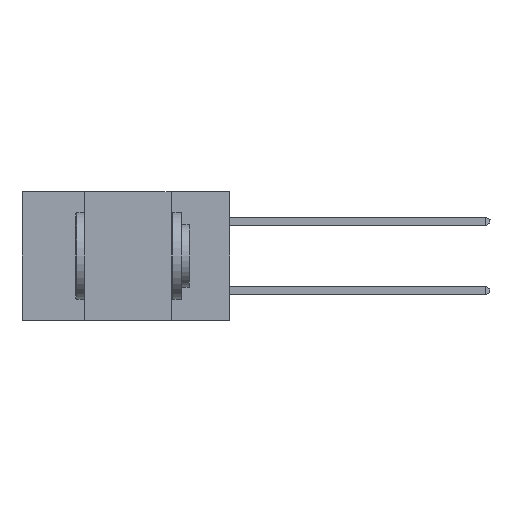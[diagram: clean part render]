
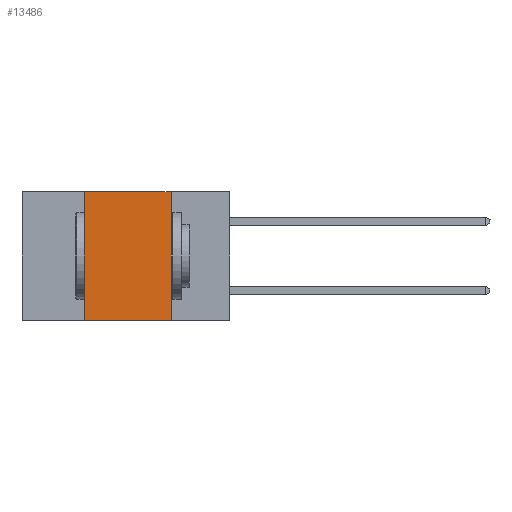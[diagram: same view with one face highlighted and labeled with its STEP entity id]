
A CAD part, left-side view. The second image highlights one B-rep face of the part: STEP entity #13486.
In plain terms, the highlighted planar face has unit normal (-1, 0, 0).
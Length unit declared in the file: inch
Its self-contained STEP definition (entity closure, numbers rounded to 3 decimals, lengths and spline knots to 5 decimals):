
#915 = LINE ( 'NONE', #7166, #13676 ) ;
#999 = FACE_OUTER_BOUND ( 'NONE', #6339, .T. ) ;
#1036 = DIRECTION ( 'NONE',  ( 0., -1., 0. ) ) ;
#2089 = DIRECTION ( 'NONE',  ( 0., 0., -1. ) ) ;
#2155 = DIRECTION ( 'NONE',  ( 1., 0., 0. ) ) ;
#2816 = VERTEX_POINT ( 'NONE', #6653 ) ;
#3292 = VECTOR ( 'NONE', #17894, 39.37008 ) ;
#3783 = EDGE_CURVE ( 'NONE', #2816, #4053, #14936, .T. ) ;
#3933 = CARTESIAN_POINT ( 'NONE',  ( 0., 0.17, 0. ) ) ;
#4053 = VERTEX_POINT ( 'NONE', #14711 ) ;
#5530 = ORIENTED_EDGE ( 'NONE', *, *, #3783, .T. ) ;
#6339 = EDGE_LOOP ( 'NONE', ( #7237, #18090, #9268, #5530 ) ) ;
#6498 = CARTESIAN_POINT ( 'NONE',  ( 0., 0.6, 0. ) ) ;
#6505 = EDGE_CURVE ( 'NONE', #9439, #10414, #10707, .T. ) ;
#6653 = CARTESIAN_POINT ( 'NONE',  ( 0., 0.42, -0.37 ) ) ;
#7166 = CARTESIAN_POINT ( 'NONE',  ( 0., 0.42, 0. ) ) ;
#7177 = LINE ( 'NONE', #18580, #16871 ) ;
#7233 = DIRECTION ( 'NONE',  ( 0., 0., 1. ) ) ;
#7237 = ORIENTED_EDGE ( 'NONE', *, *, #12607, .F. ) ;
#7510 = CARTESIAN_POINT ( 'NONE',  ( 0., 0.6, -0.37 ) ) ;
#9268 = ORIENTED_EDGE ( 'NONE', *, *, #20743, .F. ) ;
#9439 = VERTEX_POINT ( 'NONE', #13994 ) ;
#10278 = CARTESIAN_POINT ( 'NONE',  ( 0., 0.6, 0. ) ) ;
#10414 = VERTEX_POINT ( 'NONE', #3933 ) ;
#10707 = LINE ( 'NONE', #6498, #3292 ) ;
#12607 = EDGE_CURVE ( 'NONE', #10414, #4053, #7177, .T. ) ;
#13486 = ADVANCED_FACE ( 'NONE', ( #999 ), #19961, .F. ) ;
#13676 = VECTOR ( 'NONE', #7233, 39.37008 ) ;
#13994 = CARTESIAN_POINT ( 'NONE',  ( 0., 0.42, 0. ) ) ;
#14711 = CARTESIAN_POINT ( 'NONE',  ( 0., 0.17, -0.37 ) ) ;
#14936 = LINE ( 'NONE', #7510, #20038 ) ;
#15523 = DIRECTION ( 'NONE',  ( 0., 0., -1. ) ) ;
#16871 = VECTOR ( 'NONE', #2089, 39.37008 ) ;
#17894 = DIRECTION ( 'NONE',  ( 0., -1., 0. ) ) ;
#18090 = ORIENTED_EDGE ( 'NONE', *, *, #6505, .F. ) ;
#18580 = CARTESIAN_POINT ( 'NONE',  ( 0., 0.17, 0. ) ) ;
#19961 = PLANE ( 'NONE',  #20605 ) ;
#20038 = VECTOR ( 'NONE', #1036, 39.37008 ) ;
#20605 = AXIS2_PLACEMENT_3D ( 'NONE', #10278, #2155, #15523 ) ;
#20743 = EDGE_CURVE ( 'NONE', #2816, #9439, #915, .T. ) ;
